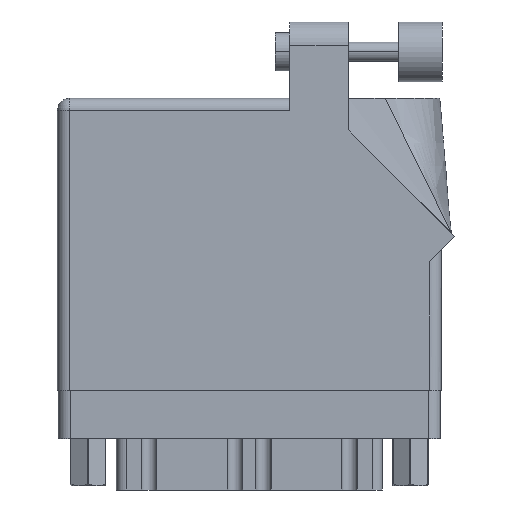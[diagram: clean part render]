
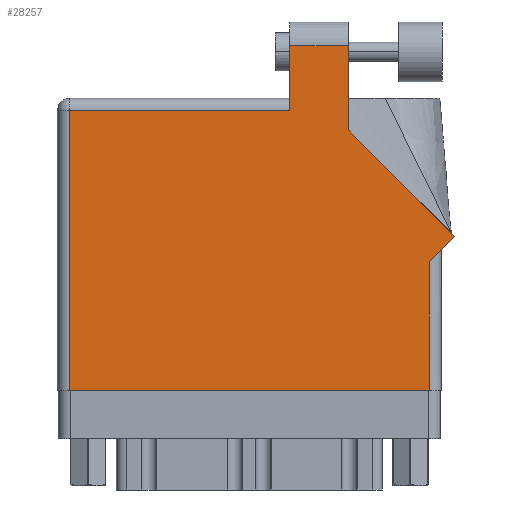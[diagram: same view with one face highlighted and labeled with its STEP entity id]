
A CAD part, front view. The second image highlights one B-rep face of the part: STEP entity #28257.
In plain terms, the highlighted face is planar.
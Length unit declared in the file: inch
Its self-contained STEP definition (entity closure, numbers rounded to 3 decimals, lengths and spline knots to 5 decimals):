
#155 = EDGE_CURVE ( 'NONE', #21332, #21715, #31474, .T. ) ;
#369 = EDGE_CURVE ( 'NONE', #41775, #33450, #43728, .T. ) ;
#947 = LINE ( 'NONE', #41862, #13598 ) ;
#2905 = DIRECTION ( 'NONE',  ( 0., -1., 0. ) ) ;
#3545 = CARTESIAN_POINT ( 'NONE',  ( 0., 0., 0. ) ) ;
#3764 = CARTESIAN_POINT ( 'NONE',  ( 0., 1.468, 0. ) ) ;
#5581 = CARTESIAN_POINT ( 'NONE',  ( 2.08071, 0.80771, 0. ) ) ;
#6198 = LINE ( 'NONE', #3545, #31794 ) ;
#7372 = EDGE_CURVE ( 'NONE', #35618, #21332, #10933, .T. ) ;
#9617 = CARTESIAN_POINT ( 'NONE',  ( 1.217, 1.805, 0. ) ) ;
#9968 = EDGE_CURVE ( 'NONE', #33450, #25331, #947, .T. ) ;
#9973 = ORIENTED_EDGE ( 'NONE', *, *, #9968, .T. ) ;
#10933 = LINE ( 'NONE', #26353, #32676 ) ;
#11576 = VECTOR ( 'NONE', #2905, 39.37008 ) ;
#13598 = VECTOR ( 'NONE', #15621, 39.37008 ) ;
#13958 = ORIENTED_EDGE ( 'NONE', *, *, #44037, .T. ) ;
#14593 = DIRECTION ( 'NONE',  ( -1., 0., 0. ) ) ;
#14702 = FACE_OUTER_BOUND ( 'NONE', #33727, .T. ) ;
#15621 = DIRECTION ( 'NONE',  ( 0., -1., 0. ) ) ;
#15751 = AXIS2_PLACEMENT_3D ( 'NONE', #29421, #41198, #18330 ) ;
#16092 = ORIENTED_EDGE ( 'NONE', *, *, #7372, .T. ) ;
#17128 = DIRECTION ( 'NONE',  ( -0.707, 0.707, 0. ) ) ;
#17521 = CARTESIAN_POINT ( 'NONE',  ( 1.217, 1.468, 0. ) ) ;
#18330 = DIRECTION ( 'NONE',  ( -1., 0., 0. ) ) ;
#18808 = PLANE ( 'NONE',  #15751 ) ;
#19781 = VECTOR ( 'NONE', #46874, 39.37008 ) ;
#20953 = VERTEX_POINT ( 'NONE', #33787 ) ;
#20969 = CARTESIAN_POINT ( 'NONE',  ( 1.217, 1.53, 0. ) ) ;
#21332 = VERTEX_POINT ( 'NONE', #46522 ) ;
#21715 = VERTEX_POINT ( 'NONE', #9617 ) ;
#25215 = CARTESIAN_POINT ( 'NONE',  ( 2.01, 0.737, 0. ) ) ;
#25331 = VERTEX_POINT ( 'NONE', #46805 ) ;
#25814 = ORIENTED_EDGE ( 'NONE', *, *, #34502, .T. ) ;
#25946 = VERTEX_POINT ( 'NONE', #26377 ) ;
#26268 = CARTESIAN_POINT ( 'NONE',  ( 0.062, 1.468, 0. ) ) ;
#26353 = CARTESIAN_POINT ( 'NONE',  ( 1.524, 1.36442, 0. ) ) ;
#26377 = CARTESIAN_POINT ( 'NONE',  ( 1.948, 0.675, 0. ) ) ;
#28257 = ADVANCED_FACE ( 'NONE', ( #14702 ), #18808, .F. ) ;
#28498 = LINE ( 'NONE', #47015, #40154 ) ;
#29174 = ORIENTED_EDGE ( 'NONE', *, *, #155, .T. ) ;
#29421 = CARTESIAN_POINT ( 'NONE',  ( 0., 1.53, 0. ) ) ;
#29799 = EDGE_CURVE ( 'NONE', #25946, #20953, #46860, .T. ) ;
#30531 = VECTOR ( 'NONE', #14593, 39.37008 ) ;
#31474 = LINE ( 'NONE', #39669, #19781 ) ;
#31794 = VECTOR ( 'NONE', #35582, 39.37008 ) ;
#32676 = VECTOR ( 'NONE', #32868, 39.37008 ) ;
#32868 = DIRECTION ( 'NONE',  ( 0., 1., 0. ) ) ;
#33362 = ORIENTED_EDGE ( 'NONE', *, *, #29799, .T. ) ;
#33450 = VERTEX_POINT ( 'NONE', #26268 ) ;
#33727 = EDGE_LOOP ( 'NONE', ( #16092, #29174, #36870, #35826, #9973, #38309, #13958, #33362, #25814 ) ) ;
#33787 = CARTESIAN_POINT ( 'NONE',  ( 2.08071, 0.80771, 0. ) ) ;
#34144 = VECTOR ( 'NONE', #43482, 39.37008 ) ;
#34382 = CARTESIAN_POINT ( 'NONE',  ( 1.948, 0., 0. ) ) ;
#34502 = EDGE_CURVE ( 'NONE', #20953, #35618, #39059, .T. ) ;
#35582 = DIRECTION ( 'NONE',  ( 1., 0., 0. ) ) ;
#35618 = VERTEX_POINT ( 'NONE', #41052 ) ;
#35826 = ORIENTED_EDGE ( 'NONE', *, *, #369, .T. ) ;
#36784 = VECTOR ( 'NONE', #17128, 39.37008 ) ;
#36870 = ORIENTED_EDGE ( 'NONE', *, *, #39502, .T. ) ;
#37513 = VERTEX_POINT ( 'NONE', #34382 ) ;
#38309 = ORIENTED_EDGE ( 'NONE', *, *, #47225, .T. ) ;
#39059 = LINE ( 'NONE', #5581, #36784 ) ;
#39502 = EDGE_CURVE ( 'NONE', #21715, #41775, #39749, .T. ) ;
#39669 = CARTESIAN_POINT ( 'NONE',  ( 1.217, 1.805, 0. ) ) ;
#39749 = LINE ( 'NONE', #20969, #11576 ) ;
#39806 = DIRECTION ( 'NONE',  ( 0., 1., 0. ) ) ;
#40154 = VECTOR ( 'NONE', #39806, 39.37008 ) ;
#41052 = CARTESIAN_POINT ( 'NONE',  ( 1.524, 1.36442, 0. ) ) ;
#41198 = DIRECTION ( 'NONE',  ( 0., 0., -1. ) ) ;
#41775 = VERTEX_POINT ( 'NONE', #17521 ) ;
#41862 = CARTESIAN_POINT ( 'NONE',  ( 0.062, 0., 0. ) ) ;
#43482 = DIRECTION ( 'NONE',  ( 0.707, 0.707, 0. ) ) ;
#43728 = LINE ( 'NONE', #3764, #30531 ) ;
#44037 = EDGE_CURVE ( 'NONE', #37513, #25946, #28498, .T. ) ;
#46522 = CARTESIAN_POINT ( 'NONE',  ( 1.524, 1.805, 0. ) ) ;
#46805 = CARTESIAN_POINT ( 'NONE',  ( 0.062, 0., 0. ) ) ;
#46860 = LINE ( 'NONE', #25215, #34144 ) ;
#46874 = DIRECTION ( 'NONE',  ( -1., 0., 0. ) ) ;
#47015 = CARTESIAN_POINT ( 'NONE',  ( 1.948, 0.737, 0. ) ) ;
#47225 = EDGE_CURVE ( 'NONE', #25331, #37513, #6198, .T. ) ;
